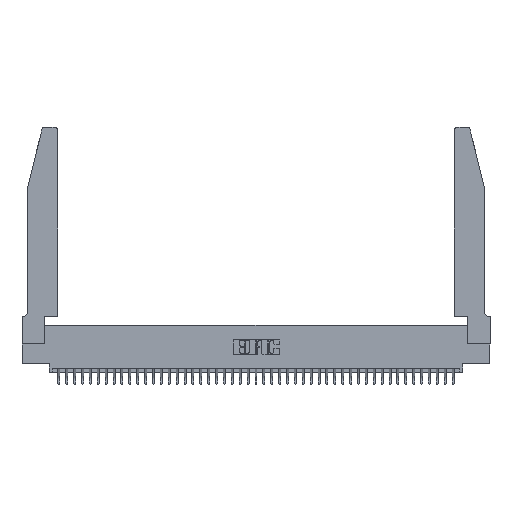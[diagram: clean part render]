
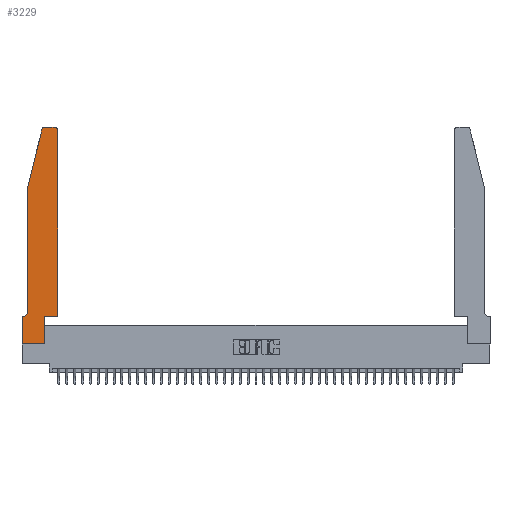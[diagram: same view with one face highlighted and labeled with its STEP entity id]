
A CAD part, top view. The second image highlights one B-rep face of the part: STEP entity #3229.
In plain terms, the highlighted planar face has unit normal (0, 0, 1).
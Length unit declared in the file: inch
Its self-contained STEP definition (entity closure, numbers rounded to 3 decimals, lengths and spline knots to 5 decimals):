
#34 = EDGE_CURVE ( 'NONE', #43604, #40679, #18099, .T. ) ;
#101 = EDGE_CURVE ( 'NONE', #40679, #24373, #38886, .T. ) ;
#261 = LINE ( 'NONE', #4595, #2934 ) ;
#276 = ORIENTED_EDGE ( 'NONE', *, *, #14082, .T. ) ;
#1264 = CIRCLE ( 'NONE', #35193, 0.03 ) ;
#1888 = VERTEX_POINT ( 'NONE', #17993 ) ;
#2815 = LINE ( 'NONE', #11091, #36844 ) ;
#2848 = ORIENTED_EDGE ( 'NONE', *, *, #24218, .T. ) ;
#2897 = LINE ( 'NONE', #42536, #16681 ) ;
#2934 = VECTOR ( 'NONE', #31376, 39.37008 ) ;
#3120 = ORIENTED_EDGE ( 'NONE', *, *, #4857, .T. ) ;
#3229 = ADVANCED_FACE ( 'NONE', ( #30621 ), #20126, .T. ) ;
#4361 = VECTOR ( 'NONE', #13729, 39.37008 ) ;
#4595 = CARTESIAN_POINT ( 'NONE',  ( 0.2865, 0.35, 0.37 ) ) ;
#4857 = EDGE_CURVE ( 'NONE', #24373, #43927, #42149, .T. ) ;
#5141 = DIRECTION ( 'NONE',  ( 0., 0., 1. ) ) ;
#5400 = VECTOR ( 'NONE', #22199, 39.37008 ) ;
#5822 = EDGE_CURVE ( 'NONE', #23021, #43604, #33094, .T. ) ;
#7653 = ORIENTED_EDGE ( 'NONE', *, *, #43398, .T. ) ;
#8747 = VERTEX_POINT ( 'NONE', #13179 ) ;
#8800 = DIRECTION ( 'NONE',  ( 0., 0., 1. ) ) ;
#11091 = CARTESIAN_POINT ( 'NONE',  ( 0.0755, 2., 0.37 ) ) ;
#11525 = CARTESIAN_POINT ( 'NONE',  ( 0.2865, 0., 0.37 ) ) ;
#12581 = CARTESIAN_POINT ( 'NONE',  ( 0.2865, 0.35, 0.37 ) ) ;
#12738 = ORIENTED_EDGE ( 'NONE', *, *, #26586, .T. ) ;
#12740 = AXIS2_PLACEMENT_3D ( 'NONE', #43013, #8800, #39872 ) ;
#12851 = DIRECTION ( 'NONE',  ( 1., 0., 0. ) ) ;
#13005 = CARTESIAN_POINT ( 'NONE',  ( 0.0755, 2., 0.37 ) ) ;
#13179 = CARTESIAN_POINT ( 'NONE',  ( 0.284, 2.75, 0.37 ) ) ;
#13721 = ORIENTED_EDGE ( 'NONE', *, *, #43649, .T. ) ;
#13729 = DIRECTION ( 'NONE',  ( 0., 1., 0. ) ) ;
#14082 = EDGE_CURVE ( 'NONE', #43927, #31666, #38914, .T. ) ;
#14383 = CARTESIAN_POINT ( 'NONE',  ( 0.0755, 0.35, 0.37 ) ) ;
#15296 = ORIENTED_EDGE ( 'NONE', *, *, #36636, .T. ) ;
#16577 = CARTESIAN_POINT ( 'NONE',  ( 0.0055, 0.35, 0.37 ) ) ;
#16681 = VECTOR ( 'NONE', #22175, 39.37008 ) ;
#16958 = ORIENTED_EDGE ( 'NONE', *, *, #42939, .T. ) ;
#17993 = CARTESIAN_POINT ( 'NONE',  ( 0.4205, 2.75, 0.37 ) ) ;
#18060 = CARTESIAN_POINT ( 'NONE',  ( 0.4505, 2.72, 0.37 ) ) ;
#18099 = CIRCLE ( 'NONE', #43646, 0.07 ) ;
#18295 = CIRCLE ( 'NONE', #12740, 0.03 ) ;
#18337 = DIRECTION ( 'NONE',  ( -1., 0., 0. ) ) ;
#18509 = ORIENTED_EDGE ( 'NONE', *, *, #34, .T. ) ;
#18790 = CARTESIAN_POINT ( 'NONE',  ( 0.0055, 0.42, 0.37 ) ) ;
#20126 = PLANE ( 'NONE',  #33497 ) ;
#20265 = LINE ( 'NONE', #34257, #4361 ) ;
#21926 = VECTOR ( 'NONE', #25276, 39.37008 ) ;
#22175 = DIRECTION ( 'NONE',  ( 1., 0., 0. ) ) ;
#22199 = DIRECTION ( 'NONE',  ( 1., 0., 0. ) ) ;
#22270 = VERTEX_POINT ( 'NONE', #31081 ) ;
#22588 = CARTESIAN_POINT ( 'NONE',  ( 0.2605, 2.75, 0.37 ) ) ;
#23021 = VERTEX_POINT ( 'NONE', #13005 ) ;
#23553 = DIRECTION ( 'NONE',  ( 0., 0., 1. ) ) ;
#24218 = EDGE_CURVE ( 'NONE', #1888, #8747, #41098, .T. ) ;
#24373 = VERTEX_POINT ( 'NONE', #36784 ) ;
#25276 = DIRECTION ( 'NONE',  ( 0., -1., 0. ) ) ;
#26259 = CARTESIAN_POINT ( 'NONE',  ( 0., 0., 0.37 ) ) ;
#26586 = EDGE_CURVE ( 'NONE', #31666, #27000, #261, .T. ) ;
#27000 = VERTEX_POINT ( 'NONE', #12581 ) ;
#28228 = DIRECTION ( 'NONE',  ( -1., 0., 0. ) ) ;
#28487 = DIRECTION ( 'NONE',  ( 0., 0., -1. ) ) ;
#28531 = DIRECTION ( 'NONE',  ( 1., 0., 0. ) ) ;
#29192 = DIRECTION ( 'NONE',  ( -1., 0., 0. ) ) ;
#30183 = CARTESIAN_POINT ( 'NONE',  ( 0.0755, 0.42, 0.37 ) ) ;
#30621 = FACE_OUTER_BOUND ( 'NONE', #32950, .T. ) ;
#30895 = DIRECTION ( 'NONE',  ( -0.239, -0.971, 0. ) ) ;
#30907 = VECTOR ( 'NONE', #39551, 39.37008 ) ;
#31081 = CARTESIAN_POINT ( 'NONE',  ( 0.25487, 2.72718, 0.37 ) ) ;
#31376 = DIRECTION ( 'NONE',  ( 0., 1., 0. ) ) ;
#31666 = VERTEX_POINT ( 'NONE', #11525 ) ;
#32568 = ORIENTED_EDGE ( 'NONE', *, *, #5822, .T. ) ;
#32738 = CARTESIAN_POINT ( 'NONE',  ( 0.0755, 2., 0.37 ) ) ;
#32950 = EDGE_LOOP ( 'NONE', ( #2848, #15296, #13721, #32568, #18509, #33991, #3120, #276, #12738, #16958, #43178, #7653 ) ) ;
#33094 = LINE ( 'NONE', #32738, #30907 ) ;
#33497 = AXIS2_PLACEMENT_3D ( 'NONE', #43922, #23553, #12851 ) ;
#33991 = ORIENTED_EDGE ( 'NONE', *, *, #101, .T. ) ;
#34257 = CARTESIAN_POINT ( 'NONE',  ( 0.4505, 0.35, 0.37 ) ) ;
#34415 = EDGE_CURVE ( 'NONE', #36635, #42352, #20265, .T. ) ;
#34640 = CARTESIAN_POINT ( 'NONE',  ( 0., 0., 0.37 ) ) ;
#35193 = AXIS2_PLACEMENT_3D ( 'NONE', #42452, #5141, #28531 ) ;
#36635 = VERTEX_POINT ( 'NONE', #43301 ) ;
#36636 = EDGE_CURVE ( 'NONE', #8747, #22270, #18295, .T. ) ;
#36784 = CARTESIAN_POINT ( 'NONE',  ( 0., 0.35, 0.37 ) ) ;
#36844 = VECTOR ( 'NONE', #30895, 39.37008 ) ;
#38886 = LINE ( 'NONE', #14383, #43133 ) ;
#38914 = LINE ( 'NONE', #42715, #5400 ) ;
#39551 = DIRECTION ( 'NONE',  ( 0., -1., 0. ) ) ;
#39872 = DIRECTION ( 'NONE',  ( 1., 0., 0. ) ) ;
#40679 = VERTEX_POINT ( 'NONE', #16577 ) ;
#41098 = LINE ( 'NONE', #22588, #42209 ) ;
#42149 = LINE ( 'NONE', #34640, #21926 ) ;
#42209 = VECTOR ( 'NONE', #29192, 39.37008 ) ;
#42352 = VERTEX_POINT ( 'NONE', #18060 ) ;
#42452 = CARTESIAN_POINT ( 'NONE',  ( 0.4205, 2.72, 0.37 ) ) ;
#42536 = CARTESIAN_POINT ( 'NONE',  ( 0.4505, 0.35, 0.37 ) ) ;
#42715 = CARTESIAN_POINT ( 'NONE',  ( 0., 0., 0.37 ) ) ;
#42939 = EDGE_CURVE ( 'NONE', #27000, #36635, #2897, .T. ) ;
#43013 = CARTESIAN_POINT ( 'NONE',  ( 0.284, 2.72, 0.37 ) ) ;
#43133 = VECTOR ( 'NONE', #28228, 39.37008 ) ;
#43178 = ORIENTED_EDGE ( 'NONE', *, *, #34415, .T. ) ;
#43301 = CARTESIAN_POINT ( 'NONE',  ( 0.4505, 0.35, 0.37 ) ) ;
#43398 = EDGE_CURVE ( 'NONE', #42352, #1888, #1264, .T. ) ;
#43604 = VERTEX_POINT ( 'NONE', #30183 ) ;
#43646 = AXIS2_PLACEMENT_3D ( 'NONE', #18790, #28487, #18337 ) ;
#43649 = EDGE_CURVE ( 'NONE', #22270, #23021, #2815, .T. ) ;
#43922 = CARTESIAN_POINT ( 'NONE',  ( 0., 0.35, 0.37 ) ) ;
#43927 = VERTEX_POINT ( 'NONE', #26259 ) ;
